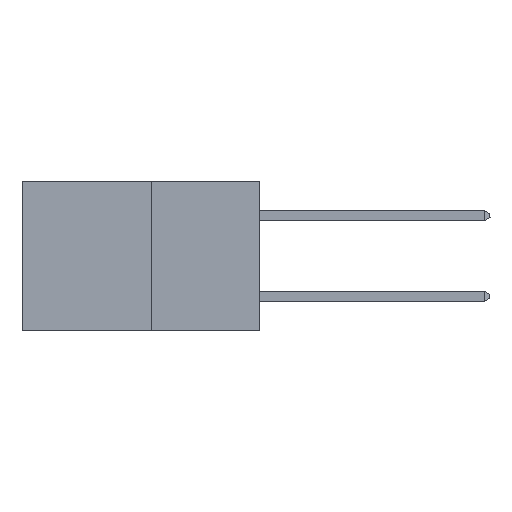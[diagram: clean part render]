
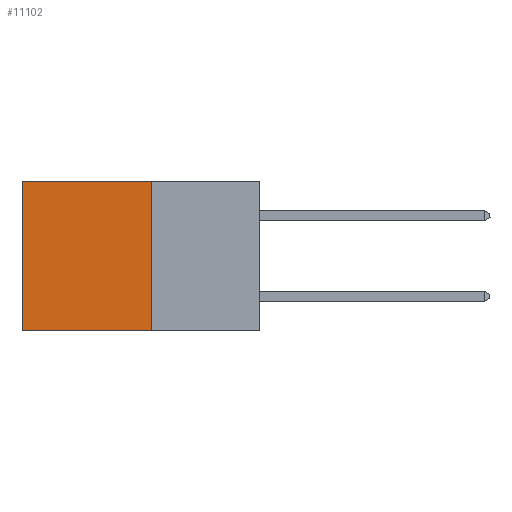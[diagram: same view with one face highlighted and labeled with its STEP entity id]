
A CAD part, left-side view. The second image highlights one B-rep face of the part: STEP entity #11102.
In plain terms, the highlighted planar face has unit normal (-1, 0, 0).
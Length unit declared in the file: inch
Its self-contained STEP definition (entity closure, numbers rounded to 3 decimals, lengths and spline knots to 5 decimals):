
#1247 = CARTESIAN_POINT ( 'NONE',  ( 0.277, 0.59, 0. ) ) ;
#1409 = DIRECTION ( 'NONE',  ( 0., 0., -1. ) ) ;
#2163 = VECTOR ( 'NONE', #12159, 39.37008 ) ;
#2714 = DIRECTION ( 'NONE',  ( 0., 0., -1. ) ) ;
#2994 = LINE ( 'NONE', #17424, #19948 ) ;
#3062 = VERTEX_POINT ( 'NONE', #1247 ) ;
#3177 = FACE_OUTER_BOUND ( 'NONE', #13449, .T. ) ;
#3720 = VERTEX_POINT ( 'NONE', #10296 ) ;
#4994 = EDGE_CURVE ( 'NONE', #3062, #3720, #15312, .T. ) ;
#5222 = AXIS2_PLACEMENT_3D ( 'NONE', #7616, #12600, #2714 ) ;
#5488 = LINE ( 'NONE', #19460, #13734 ) ;
#7616 = CARTESIAN_POINT ( 'NONE',  ( 0.277, 0.27, -0.37 ) ) ;
#7732 = ORIENTED_EDGE ( 'NONE', *, *, #11218, .F. ) ;
#9057 = EDGE_CURVE ( 'NONE', #12102, #3720, #2994, .T. ) ;
#9541 = EDGE_CURVE ( 'NONE', #13750, #3062, #15590, .T. ) ;
#10296 = CARTESIAN_POINT ( 'NONE',  ( 0.277, 0.59, -0.37 ) ) ;
#10685 = VECTOR ( 'NONE', #18191, 39.37008 ) ;
#11102 = ADVANCED_FACE ( 'NONE', ( #3177 ), #15819, .F. ) ;
#11218 = EDGE_CURVE ( 'NONE', #13750, #12102, #5488, .T. ) ;
#12102 = VERTEX_POINT ( 'NONE', #14928 ) ;
#12159 = DIRECTION ( 'NONE',  ( 0., 0., -1. ) ) ;
#12600 = DIRECTION ( 'NONE',  ( 1., 0., 0. ) ) ;
#13449 = EDGE_LOOP ( 'NONE', ( #16307, #16775, #7732, #18303 ) ) ;
#13734 = VECTOR ( 'NONE', #1409, 39.37008 ) ;
#13750 = VERTEX_POINT ( 'NONE', #20287 ) ;
#14928 = CARTESIAN_POINT ( 'NONE',  ( 0.277, 0.27, -0.37 ) ) ;
#15312 = LINE ( 'NONE', #16031, #2163 ) ;
#15590 = LINE ( 'NONE', #16165, #10685 ) ;
#15819 = PLANE ( 'NONE',  #5222 ) ;
#16031 = CARTESIAN_POINT ( 'NONE',  ( 0.277, 0.59, -0.37 ) ) ;
#16165 = CARTESIAN_POINT ( 'NONE',  ( 0.277, 0.27, 0. ) ) ;
#16307 = ORIENTED_EDGE ( 'NONE', *, *, #4994, .T. ) ;
#16775 = ORIENTED_EDGE ( 'NONE', *, *, #9057, .F. ) ;
#17424 = CARTESIAN_POINT ( 'NONE',  ( 0.277, 0.27, -0.37 ) ) ;
#17568 = DIRECTION ( 'NONE',  ( 0., 1., 0. ) ) ;
#18191 = DIRECTION ( 'NONE',  ( 0., 1., 0. ) ) ;
#18303 = ORIENTED_EDGE ( 'NONE', *, *, #9541, .T. ) ;
#19460 = CARTESIAN_POINT ( 'NONE',  ( 0.277, 0.27, -0.37 ) ) ;
#19948 = VECTOR ( 'NONE', #17568, 39.37008 ) ;
#20287 = CARTESIAN_POINT ( 'NONE',  ( 0.277, 0.27, 0. ) ) ;
